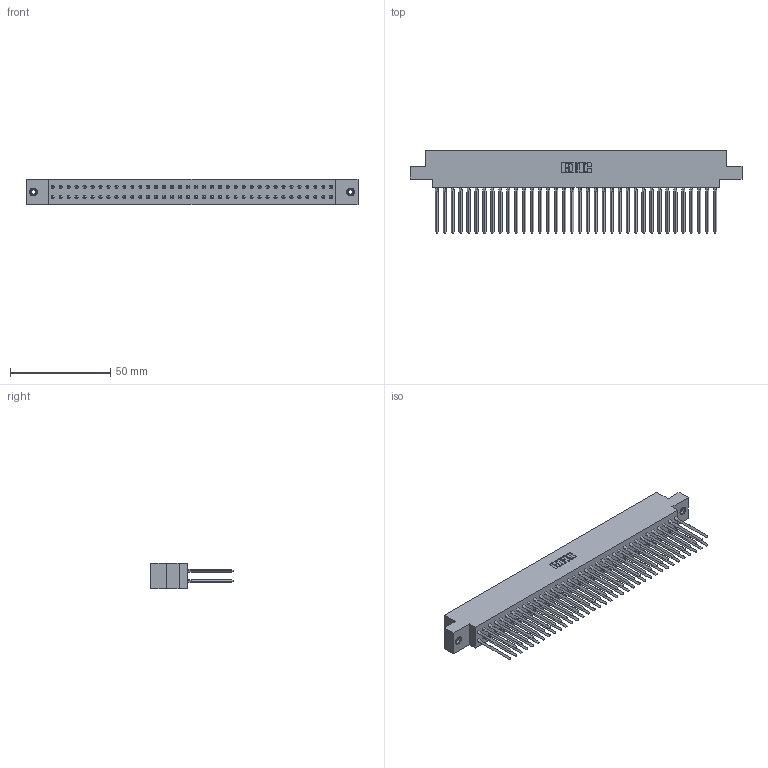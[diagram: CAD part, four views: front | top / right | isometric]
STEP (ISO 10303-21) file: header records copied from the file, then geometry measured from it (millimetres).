
FILE_DESCRIPTION (( 'STEP AP203' ), '1' );
FILE_NAME ('317-072-543-808.STEP', '2020-02-28T07:43:56', ( '' ), ( '' ), 'SwSTEP 2.0', 'SolidWorks 2016', '' );
FILE_SCHEMA (( 'CONFIG_CONTROL_DESIGN' ));
Length unit declared in the file: inch
Products named in the file (4): 317 Part_.156 Dia - TI; 317-072-543-808; 345-250-001_345-250-003-102; 317-290-001_543
Assembly tree (75 placements, depth 2):
  317-072-543-808
    317 Part_.156 Dia - TI
    317-290-001_543  x72
    345-250-001_345-250-003-102  x2
Bounding box: 165.35 x 41.15 x 12.7 mm (x, y, z)
Volume: 27900.5 mm3; surface area: 42112.7 mm2
Topology: 75 solids, 75 shells, 6570 faces, 18195 edges, 11714 vertices
Faces by surface type: plane 5346, cylinder 920, bspline 288, cone 12, torus 4
Entity records: 54061 total; most frequent: CARTESIAN_POINT 9818, ORIENTED_EDGE 9310, DIRECTION 7807, EDGE_CURVE 4655, VECTOR 4379, LINE 4379, VERTEX_POINT 3093, AXIS2_PLACEMENT_3D 1714
